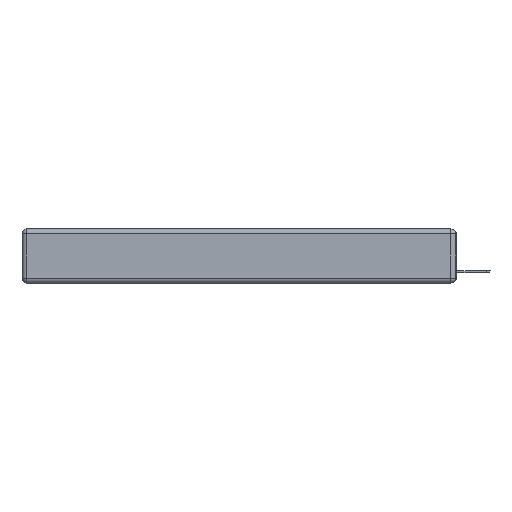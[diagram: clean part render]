
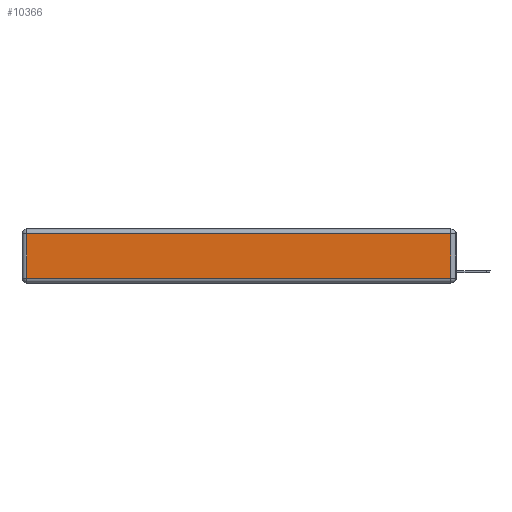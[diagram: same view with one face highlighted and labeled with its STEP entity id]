
A CAD part, left-side view. The second image highlights one B-rep face of the part: STEP entity #10366.
In plain terms, the highlighted planar face has unit normal (-1, 0, 0).
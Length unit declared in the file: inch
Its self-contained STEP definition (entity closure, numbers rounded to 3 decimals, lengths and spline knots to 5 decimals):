
#167 = VERTEX_POINT ( 'NONE', #6872 ) ;
#613 = EDGE_CURVE ( 'NONE', #167, #11324, #10601, .T. ) ;
#708 = DIRECTION ( 'NONE',  ( 0., 0., -1. ) ) ;
#832 = CARTESIAN_POINT ( 'NONE',  ( 0., 2.72, -0.313 ) ) ;
#1437 = LINE ( 'NONE', #1778, #14429 ) ;
#1778 = CARTESIAN_POINT ( 'NONE',  ( 0., 2.72, -0.343 ) ) ;
#3370 = ORIENTED_EDGE ( 'NONE', *, *, #613, .T. ) ;
#4505 = DIRECTION ( 'NONE',  ( 0., -1., 0. ) ) ;
#4910 = VECTOR ( 'NONE', #8253, 39.37008 ) ;
#5115 = CARTESIAN_POINT ( 'NONE',  ( 0., 0., -0.343 ) ) ;
#5394 = ORIENTED_EDGE ( 'NONE', *, *, #11652, .T. ) ;
#5521 = EDGE_LOOP ( 'NONE', ( #5394, #3370, #7778, #10139 ) ) ;
#6872 = CARTESIAN_POINT ( 'NONE',  ( 0., 0.03, -0.313 ) ) ;
#7178 = FACE_OUTER_BOUND ( 'NONE', #5521, .T. ) ;
#7532 = EDGE_CURVE ( 'NONE', #11513, #13551, #1437, .T. ) ;
#7610 = VECTOR ( 'NONE', #14267, 39.37008 ) ;
#7778 = ORIENTED_EDGE ( 'NONE', *, *, #13890, .T. ) ;
#7966 = CARTESIAN_POINT ( 'NONE',  ( 0., 0.03, -0.03 ) ) ;
#7999 = VECTOR ( 'NONE', #4505, 39.37008 ) ;
#8253 = DIRECTION ( 'NONE',  ( 0., 1., 0. ) ) ;
#9652 = PLANE ( 'NONE',  #12504 ) ;
#9696 = DIRECTION ( 'NONE',  ( -1., 0., 0. ) ) ;
#10031 = CARTESIAN_POINT ( 'NONE',  ( 0., 0., -0.313 ) ) ;
#10139 = ORIENTED_EDGE ( 'NONE', *, *, #7532, .T. ) ;
#10358 = LINE ( 'NONE', #10630, #4910 ) ;
#10366 = ADVANCED_FACE ( 'NONE', ( #7178 ), #9652, .T. ) ;
#10601 = LINE ( 'NONE', #11979, #7610 ) ;
#10630 = CARTESIAN_POINT ( 'NONE',  ( 0., 2.75, -0.03 ) ) ;
#11027 = CARTESIAN_POINT ( 'NONE',  ( 0., 2.72, -0.03 ) ) ;
#11324 = VERTEX_POINT ( 'NONE', #7966 ) ;
#11513 = VERTEX_POINT ( 'NONE', #11027 ) ;
#11652 = EDGE_CURVE ( 'NONE', #13551, #167, #14317, .T. ) ;
#11979 = CARTESIAN_POINT ( 'NONE',  ( 0., 0.03, -0.343 ) ) ;
#12504 = AXIS2_PLACEMENT_3D ( 'NONE', #5115, #9696, #14118 ) ;
#13551 = VERTEX_POINT ( 'NONE', #832 ) ;
#13890 = EDGE_CURVE ( 'NONE', #11324, #11513, #10358, .T. ) ;
#14118 = DIRECTION ( 'NONE',  ( 0., 0., 1. ) ) ;
#14267 = DIRECTION ( 'NONE',  ( 0., 0., 1. ) ) ;
#14317 = LINE ( 'NONE', #10031, #7999 ) ;
#14429 = VECTOR ( 'NONE', #708, 39.37008 ) ;
